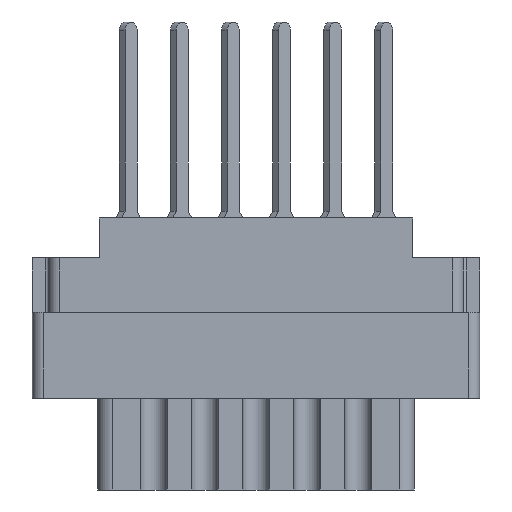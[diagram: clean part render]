
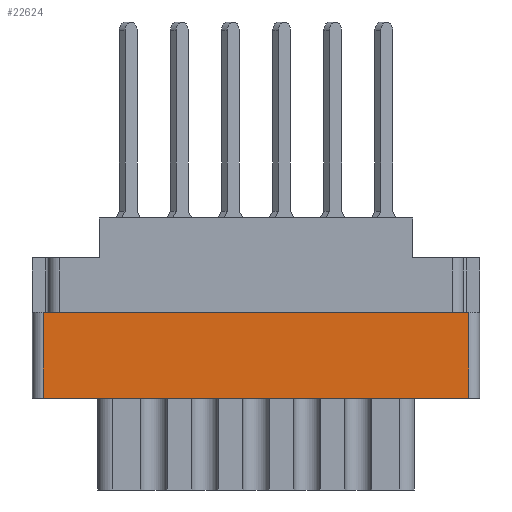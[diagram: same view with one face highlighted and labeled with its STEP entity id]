
A CAD part, front view. The second image highlights one B-rep face of the part: STEP entity #22624.
In plain terms, the highlighted planar face has unit normal (0, -1, 0).
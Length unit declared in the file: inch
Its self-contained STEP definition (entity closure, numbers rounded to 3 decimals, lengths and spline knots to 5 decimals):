
#443 = VECTOR ( 'NONE', #15841, 39.37008 ) ;
#482 = AXIS2_PLACEMENT_3D ( 'NONE', #2094, #17012, #22265 ) ;
#1171 = ORIENTED_EDGE ( 'NONE', *, *, #11928, .T. ) ;
#1830 = ORIENTED_EDGE ( 'NONE', *, *, #5778, .F. ) ;
#2094 = CARTESIAN_POINT ( 'NONE',  ( -0.624, -0.343, -0.798 ) ) ;
#2839 = CARTESIAN_POINT ( 'NONE',  ( -0.656, -0.343, -0.277 ) ) ;
#3179 = DIRECTION ( 'NONE',  ( -1., 0., 0. ) ) ;
#3461 = VECTOR ( 'NONE', #16588, 39.37008 ) ;
#4865 = VERTEX_POINT ( 'NONE', #6712 ) ;
#5108 = CARTESIAN_POINT ( 'NONE',  ( 0.624, -0.343, -0.277 ) ) ;
#5304 = VERTEX_POINT ( 'NONE', #5108 ) ;
#5778 = EDGE_CURVE ( 'NONE', #22657, #4865, #19420, .T. ) ;
#6712 = CARTESIAN_POINT ( 'NONE',  ( -0.624, -0.343, -0.529 ) ) ;
#8598 = VECTOR ( 'NONE', #3179, 39.37008 ) ;
#8619 = CARTESIAN_POINT ( 'NONE',  ( -0.624, -0.343, -0.277 ) ) ;
#8868 = ORIENTED_EDGE ( 'NONE', *, *, #22758, .F. ) ;
#10329 = DIRECTION ( 'NONE',  ( 0., 0., 1. ) ) ;
#11077 = EDGE_CURVE ( 'NONE', #20488, #5304, #12147, .T. ) ;
#11928 = EDGE_CURVE ( 'NONE', #22657, #5304, #22184, .T. ) ;
#12147 = LINE ( 'NONE', #2839, #443 ) ;
#12349 = VECTOR ( 'NONE', #10329, 39.37008 ) ;
#12961 = FACE_OUTER_BOUND ( 'NONE', #22297, .T. ) ;
#14984 = CARTESIAN_POINT ( 'NONE',  ( 0.624, -0.343, -0.529 ) ) ;
#15841 = DIRECTION ( 'NONE',  ( 1., 0., 0. ) ) ;
#16588 = DIRECTION ( 'NONE',  ( 0., 0., 1. ) ) ;
#17012 = DIRECTION ( 'NONE',  ( 0., -1., 0. ) ) ;
#17309 = ORIENTED_EDGE ( 'NONE', *, *, #11077, .F. ) ;
#18374 = CARTESIAN_POINT ( 'NONE',  ( 0.624, -0.343, -0.798 ) ) ;
#19420 = LINE ( 'NONE', #21435, #8598 ) ;
#20134 = PLANE ( 'NONE',  #482 ) ;
#20488 = VERTEX_POINT ( 'NONE', #8619 ) ;
#20705 = LINE ( 'NONE', #21181, #12349 ) ;
#21181 = CARTESIAN_POINT ( 'NONE',  ( -0.624, -0.343, -0.798 ) ) ;
#21435 = CARTESIAN_POINT ( 'NONE',  ( 0.624, -0.343, -0.529 ) ) ;
#22184 = LINE ( 'NONE', #18374, #3461 ) ;
#22265 = DIRECTION ( 'NONE',  ( 0., 0., -1. ) ) ;
#22297 = EDGE_LOOP ( 'NONE', ( #8868, #1830, #1171, #17309 ) ) ;
#22624 = ADVANCED_FACE ( 'NONE', ( #12961 ), #20134, .T. ) ;
#22657 = VERTEX_POINT ( 'NONE', #14984 ) ;
#22758 = EDGE_CURVE ( 'NONE', #4865, #20488, #20705, .T. ) ;
